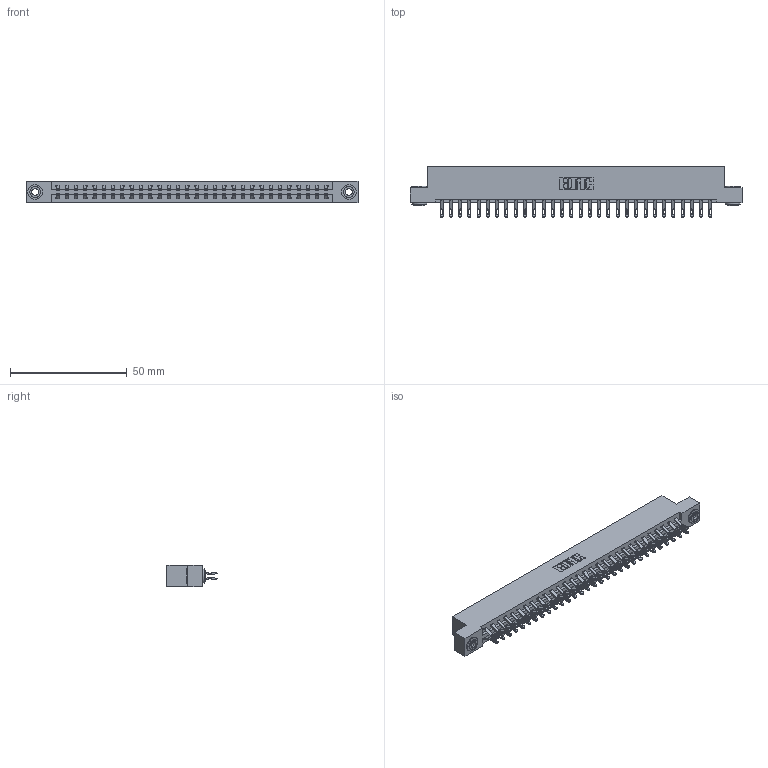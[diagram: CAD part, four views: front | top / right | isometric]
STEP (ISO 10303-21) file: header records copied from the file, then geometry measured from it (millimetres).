
FILE_DESCRIPTION (( 'STEP AP203' ), '1' );
FILE_NAME ('337-060-555-203.STEP', '2019-10-09T20:40:54', ( '' ), ( '' ), 'SwSTEP 2.0', 'SolidWorks 2016', '' );
FILE_SCHEMA (( 'CONFIG_CONTROL_DESIGN' ));
Length unit declared in the file: inch
Products named in the file (4): 337-060-555-203; 337 Part_Flush Mounting Lugs - 0.156 Dia-TH; 345-250-002_345-250-002-102; 345-292-001_555 Tail
Assembly tree (63 placements, depth 2):
  337-060-555-203
    337 Part_Flush Mounting Lugs - 0.156 Dia-TH
    345-292-001_555 Tail  x60
    345-250-002_345-250-002-102  x2
Bounding box: 141.88 x 21.47 x 9.4 mm (x, y, z)
Volume: 14986.6 mm3; surface area: 17706.1 mm2
Topology: 63 solids, 63 shells, 3752 faces, 11727 edges, 7814 vertices
Faces by surface type: plane 2240, cylinder 1504, cone 8
Entity records: 25788 total; most frequent: CARTESIAN_POINT 4363, ORIENTED_EDGE 4262, DIRECTION 3737, EDGE_CURVE 2131, VECTOR 1959, LINE 1959, VERTEX_POINT 1418, AXIS2_PLACEMENT_3D 889
